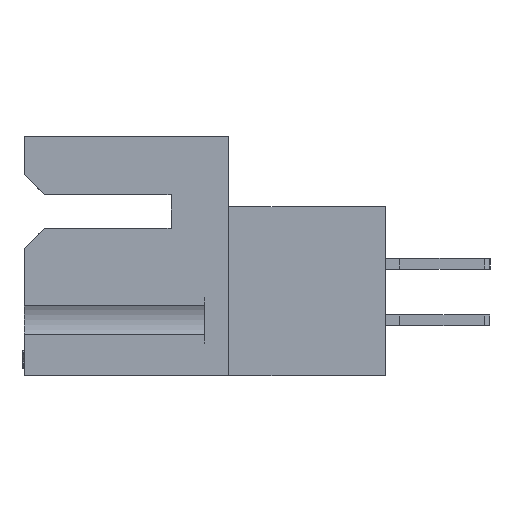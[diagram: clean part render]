
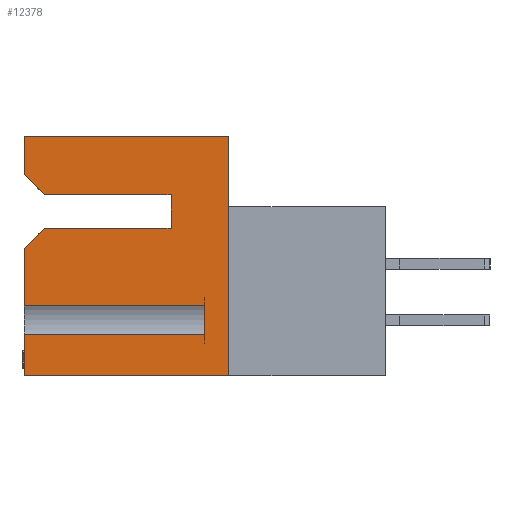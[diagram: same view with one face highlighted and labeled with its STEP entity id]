
A CAD part, left-side view. The second image highlights one B-rep face of the part: STEP entity #12378.
In plain terms, the highlighted planar face has unit normal (-1, 0, 0).
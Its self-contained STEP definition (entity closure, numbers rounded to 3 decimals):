
#124 = VERTEX_POINT ( 'NONE', #18287 ) ;
#199 = EDGE_CURVE ( 'NONE', #27401, #1840, #27749, .T. ) ;
#1108 = VECTOR ( 'NONE', #27213, 1000. ) ;
#1653 = ORIENTED_EDGE ( 'NONE', *, *, #17850, .T. ) ;
#1840 = VERTEX_POINT ( 'NONE', #38895 ) ;
#1857 = VERTEX_POINT ( 'NONE', #31479 ) ;
#1883 = CARTESIAN_POINT ( 'NONE',  ( 0., 11.506, -13.487 ) ) ;
#2496 = AXIS2_PLACEMENT_3D ( 'NONE', #4781, #26234, #26072 ) ;
#3403 = CARTESIAN_POINT ( 'NONE',  ( 0., 3.251, -3.302 ) ) ;
#4781 = CARTESIAN_POINT ( 'NONE',  ( 0., 0., 0. ) ) ;
#5419 = VECTOR ( 'NONE', #26179, 1000. ) ;
#6029 = VERTEX_POINT ( 'NONE', #41353 ) ;
#6097 = CARTESIAN_POINT ( 'NONE',  ( 0., 11.506, -9.556 ) ) ;
#6675 = LINE ( 'NONE', #27302, #17263 ) ;
#6785 = VECTOR ( 'NONE', #31670, 1000. ) ;
#6799 = ORIENTED_EDGE ( 'NONE', *, *, #199, .F. ) ;
#7162 = EDGE_CURVE ( 'NONE', #1840, #11272, #6675, .T. ) ;
#7197 = VECTOR ( 'NONE', #34269, 1000. ) ;
#7413 = CARTESIAN_POINT ( 'NONE',  ( 0., 1.346, -11.17 ) ) ;
#7485 = CARTESIAN_POINT ( 'NONE',  ( 0., 1.346, 0. ) ) ;
#7898 = LINE ( 'NONE', #7485, #6785 ) ;
#8121 = LINE ( 'NONE', #36880, #11467 ) ;
#8571 = VECTOR ( 'NONE', #42271, 1000. ) ;
#11272 = VERTEX_POINT ( 'NONE', #3403 ) ;
#11467 = VECTOR ( 'NONE', #11629, 1000. ) ;
#11629 = DIRECTION ( 'NONE',  ( 0., 0., -1. ) ) ;
#11673 = LINE ( 'NONE', #41265, #1108 ) ;
#11906 = ORIENTED_EDGE ( 'NONE', *, *, #40482, .T. ) ;
#12055 = VERTEX_POINT ( 'NONE', #36960 ) ;
#12378 = ADVANCED_FACE ( 'NONE', ( #36656 ), #33776, .F. ) ;
#12590 = VECTOR ( 'NONE', #12703, 1000. ) ;
#12703 = DIRECTION ( 'NONE',  ( 0., 0.707, -0.707 ) ) ;
#12737 = VECTOR ( 'NONE', #40234, 1000. ) ;
#13414 = VERTEX_POINT ( 'NONE', #31530 ) ;
#13719 = LINE ( 'NONE', #33796, #12590 ) ;
#14313 = ORIENTED_EDGE ( 'NONE', *, *, #15924, .F. ) ;
#14881 = DIRECTION ( 'NONE',  ( 0., -1., 0. ) ) ;
#15397 = DIRECTION ( 'NONE',  ( 0., 1., 0. ) ) ;
#15899 = VERTEX_POINT ( 'NONE', #1883 ) ;
#15924 = EDGE_CURVE ( 'NONE', #15899, #124, #20052, .T. ) ;
#15996 = EDGE_CURVE ( 'NONE', #34068, #1857, #11673, .T. ) ;
#17263 = VECTOR ( 'NONE', #30818, 1000. ) ;
#17822 = DIRECTION ( 'NONE',  ( 0., -1., 0. ) ) ;
#17850 = EDGE_CURVE ( 'NONE', #27401, #1857, #13719, .T. ) ;
#18035 = CARTESIAN_POINT ( 'NONE',  ( 0., 11.506, -13.487 ) ) ;
#18271 = ORIENTED_EDGE ( 'NONE', *, *, #7162, .F. ) ;
#18287 = CARTESIAN_POINT ( 'NONE',  ( 0., 11.506, -11.17 ) ) ;
#19255 = LINE ( 'NONE', #18035, #40297 ) ;
#19350 = CARTESIAN_POINT ( 'NONE',  ( 0., 1.346, -9.556 ) ) ;
#19626 = VERTEX_POINT ( 'NONE', #7413 ) ;
#20052 = LINE ( 'NONE', #34434, #7197 ) ;
#21235 = CARTESIAN_POINT ( 'NONE',  ( 0., 1.346, -11.17 ) ) ;
#21355 = CARTESIAN_POINT ( 'NONE',  ( 0., 0., 0. ) ) ;
#21740 = CARTESIAN_POINT ( 'NONE',  ( 0., 11.506, 0. ) ) ;
#23062 = EDGE_CURVE ( 'NONE', #19626, #33797, #7898, .T. ) ;
#23310 = ORIENTED_EDGE ( 'NONE', *, *, #41894, .F. ) ;
#24619 = DIRECTION ( 'NONE',  ( 0., 1., 0. ) ) ;
#25596 = ORIENTED_EDGE ( 'NONE', *, *, #36269, .F. ) ;
#25687 = VECTOR ( 'NONE', #24619, 1000. ) ;
#26072 = DIRECTION ( 'NONE',  ( 0., 0., -1. ) ) ;
#26179 = DIRECTION ( 'NONE',  ( 0., -0.707, -0.707 ) ) ;
#26208 = ORIENTED_EDGE ( 'NONE', *, *, #43590, .F. ) ;
#26234 = DIRECTION ( 'NONE',  ( 1., 0., 0. ) ) ;
#26634 = VECTOR ( 'NONE', #17822, 1000. ) ;
#27213 = DIRECTION ( 'NONE',  ( 0., 0., 1. ) ) ;
#27302 = CARTESIAN_POINT ( 'NONE',  ( 0., 3.251, -5.182 ) ) ;
#27401 = VERTEX_POINT ( 'NONE', #39623 ) ;
#27492 = EDGE_CURVE ( 'NONE', #12055, #6029, #37571, .T. ) ;
#27749 = LINE ( 'NONE', #38991, #26634 ) ;
#28608 = EDGE_CURVE ( 'NONE', #12055, #13414, #19255, .T. ) ;
#28622 = LINE ( 'NONE', #28899, #36889 ) ;
#28698 = CARTESIAN_POINT ( 'NONE',  ( 0., 0., -13.487 ) ) ;
#28899 = CARTESIAN_POINT ( 'NONE',  ( 0., 0., -3.302 ) ) ;
#29193 = EDGE_CURVE ( 'NONE', #13414, #35188, #44272, .T. ) ;
#29211 = VERTEX_POINT ( 'NONE', #28698 ) ;
#30818 = DIRECTION ( 'NONE',  ( 0., 0., 1. ) ) ;
#31479 = CARTESIAN_POINT ( 'NONE',  ( 0., 11.506, -6.325 ) ) ;
#31530 = CARTESIAN_POINT ( 'NONE',  ( 0., 11.506, 0. ) ) ;
#31587 = ORIENTED_EDGE ( 'NONE', *, *, #29193, .F. ) ;
#31670 = DIRECTION ( 'NONE',  ( 0., 0., 1. ) ) ;
#33776 = PLANE ( 'NONE',  #2496 ) ;
#33796 = CARTESIAN_POINT ( 'NONE',  ( 0., 10.363, -5.182 ) ) ;
#33797 = VERTEX_POINT ( 'NONE', #40606 ) ;
#34068 = VERTEX_POINT ( 'NONE', #6097 ) ;
#34269 = DIRECTION ( 'NONE',  ( 0., 0., 1. ) ) ;
#34434 = CARTESIAN_POINT ( 'NONE',  ( 0., 11.506, -13.487 ) ) ;
#34929 = ORIENTED_EDGE ( 'NONE', *, *, #43122, .T. ) ;
#35104 = CARTESIAN_POINT ( 'NONE',  ( 0., -8.814, -13.487 ) ) ;
#35188 = VERTEX_POINT ( 'NONE', #21355 ) ;
#36044 = LINE ( 'NONE', #19350, #12737 ) ;
#36269 = EDGE_CURVE ( 'NONE', #35188, #29211, #8121, .T. ) ;
#36656 = FACE_OUTER_BOUND ( 'NONE', #44013, .T. ) ;
#36880 = CARTESIAN_POINT ( 'NONE',  ( 0., 0., 0. ) ) ;
#36889 = VECTOR ( 'NONE', #15397, 1000. ) ;
#36960 = CARTESIAN_POINT ( 'NONE',  ( 0., 11.506, -2.159 ) ) ;
#37370 = LINE ( 'NONE', #21235, #8571 ) ;
#37554 = ORIENTED_EDGE ( 'NONE', *, *, #15996, .F. ) ;
#37571 = LINE ( 'NONE', #40712, #5419 ) ;
#37866 = ORIENTED_EDGE ( 'NONE', *, *, #28608, .F. ) ;
#38733 = VECTOR ( 'NONE', #14881, 1000. ) ;
#38895 = CARTESIAN_POINT ( 'NONE',  ( 0., 3.251, -5.182 ) ) ;
#38991 = CARTESIAN_POINT ( 'NONE',  ( 0., 0., -5.182 ) ) ;
#39553 = ORIENTED_EDGE ( 'NONE', *, *, #23062, .F. ) ;
#39623 = CARTESIAN_POINT ( 'NONE',  ( 0., 10.363, -5.182 ) ) ;
#40234 = DIRECTION ( 'NONE',  ( 0., -1., 0. ) ) ;
#40297 = VECTOR ( 'NONE', #42935, 1000. ) ;
#40482 = EDGE_CURVE ( 'NONE', #19626, #124, #37370, .T. ) ;
#40606 = CARTESIAN_POINT ( 'NONE',  ( 0., 1.346, -9.556 ) ) ;
#40656 = LINE ( 'NONE', #35104, #25687 ) ;
#40712 = CARTESIAN_POINT ( 'NONE',  ( 0., 10.363, -3.302 ) ) ;
#41221 = ORIENTED_EDGE ( 'NONE', *, *, #27492, .T. ) ;
#41265 = CARTESIAN_POINT ( 'NONE',  ( 0., 11.506, -13.487 ) ) ;
#41353 = CARTESIAN_POINT ( 'NONE',  ( 0., 10.363, -3.302 ) ) ;
#41894 = EDGE_CURVE ( 'NONE', #29211, #15899, #40656, .T. ) ;
#42271 = DIRECTION ( 'NONE',  ( 0., 1., 0. ) ) ;
#42935 = DIRECTION ( 'NONE',  ( 0., 0., 1. ) ) ;
#43122 = EDGE_CURVE ( 'NONE', #34068, #33797, #36044, .T. ) ;
#43590 = EDGE_CURVE ( 'NONE', #11272, #6029, #28622, .T. ) ;
#44013 = EDGE_LOOP ( 'NONE', ( #23310, #25596, #31587, #37866, #41221, #26208, #18271, #6799, #1653, #37554, #34929, #39553, #11906, #14313 ) ) ;
#44272 = LINE ( 'NONE', #21740, #38733 ) ;
